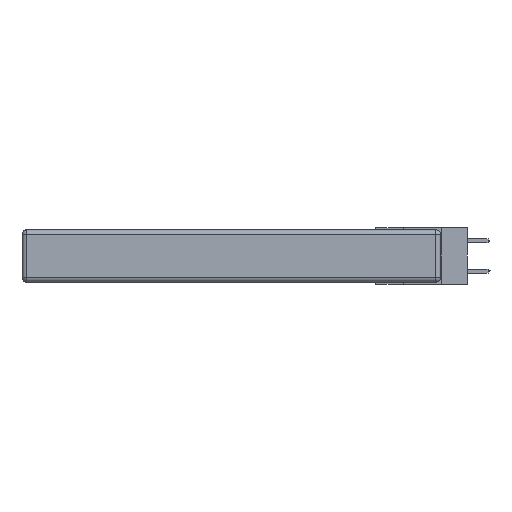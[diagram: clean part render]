
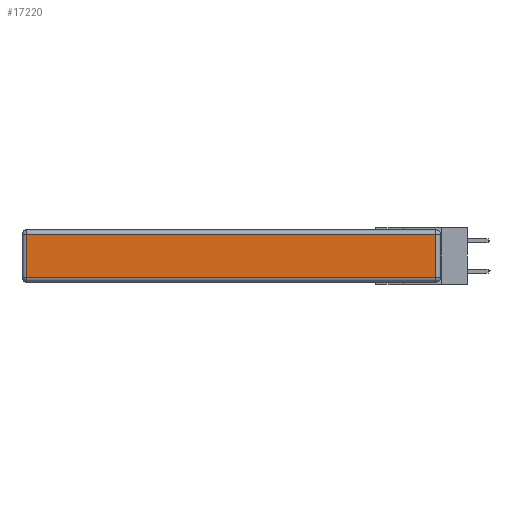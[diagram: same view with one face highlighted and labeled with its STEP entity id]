
A CAD part, left-side view. The second image highlights one B-rep face of the part: STEP entity #17220.
In plain terms, the highlighted planar face has unit normal (-1, 0, 0).
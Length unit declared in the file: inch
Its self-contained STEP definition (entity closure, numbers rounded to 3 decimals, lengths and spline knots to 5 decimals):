
#131 = LINE ( 'NONE', #1619, #1203 ) ;
#206 = CARTESIAN_POINT ( 'NONE',  ( 0., 0., -0.313 ) ) ;
#222 = LINE ( 'NONE', #6790, #11490 ) ;
#1203 = VECTOR ( 'NONE', #11000, 39.37008 ) ;
#1533 = VERTEX_POINT ( 'NONE', #15510 ) ;
#1619 = CARTESIAN_POINT ( 'NONE',  ( 0., 2.75, -0.03 ) ) ;
#1954 = EDGE_CURVE ( 'NONE', #11402, #1533, #14705, .T. ) ;
#1994 = FACE_OUTER_BOUND ( 'NONE', #16047, .T. ) ;
#2025 = LINE ( 'NONE', #206, #3894 ) ;
#3308 = EDGE_CURVE ( 'NONE', #15750, #4034, #222, .T. ) ;
#3894 = VECTOR ( 'NONE', #5530, 39.37008 ) ;
#4034 = VERTEX_POINT ( 'NONE', #7502 ) ;
#4145 = VECTOR ( 'NONE', #9878, 39.37008 ) ;
#5096 = DIRECTION ( 'NONE',  ( 0., 0., 1. ) ) ;
#5530 = DIRECTION ( 'NONE',  ( 0., -1., 0. ) ) ;
#5720 = AXIS2_PLACEMENT_3D ( 'NONE', #16996, #17112, #5096 ) ;
#6790 = CARTESIAN_POINT ( 'NONE',  ( 0., 2.72, -0.343 ) ) ;
#7502 = CARTESIAN_POINT ( 'NONE',  ( 0., 2.72, -0.313 ) ) ;
#7519 = ORIENTED_EDGE ( 'NONE', *, *, #1954, .T. ) ;
#7670 = PLANE ( 'NONE',  #5720 ) ;
#7780 = EDGE_CURVE ( 'NONE', #1533, #15750, #131, .T. ) ;
#8130 = EDGE_CURVE ( 'NONE', #4034, #11402, #2025, .T. ) ;
#9878 = DIRECTION ( 'NONE',  ( 0., 0., 1. ) ) ;
#11000 = DIRECTION ( 'NONE',  ( 0., 1., 0. ) ) ;
#11402 = VERTEX_POINT ( 'NONE', #16280 ) ;
#11416 = CARTESIAN_POINT ( 'NONE',  ( 0., 0.03, -0.343 ) ) ;
#11490 = VECTOR ( 'NONE', #15098, 39.37008 ) ;
#14193 = CARTESIAN_POINT ( 'NONE',  ( 0., 2.72, -0.03 ) ) ;
#14705 = LINE ( 'NONE', #11416, #4145 ) ;
#15098 = DIRECTION ( 'NONE',  ( 0., 0., -1. ) ) ;
#15510 = CARTESIAN_POINT ( 'NONE',  ( 0., 0.03, -0.03 ) ) ;
#15656 = ORIENTED_EDGE ( 'NONE', *, *, #3308, .T. ) ;
#15750 = VERTEX_POINT ( 'NONE', #14193 ) ;
#16047 = EDGE_LOOP ( 'NONE', ( #16347, #7519, #16743, #15656 ) ) ;
#16280 = CARTESIAN_POINT ( 'NONE',  ( 0., 0.03, -0.313 ) ) ;
#16347 = ORIENTED_EDGE ( 'NONE', *, *, #8130, .T. ) ;
#16743 = ORIENTED_EDGE ( 'NONE', *, *, #7780, .T. ) ;
#16996 = CARTESIAN_POINT ( 'NONE',  ( 0., 0., -0.343 ) ) ;
#17112 = DIRECTION ( 'NONE',  ( -1., 0., 0. ) ) ;
#17220 = ADVANCED_FACE ( 'NONE', ( #1994 ), #7670, .T. ) ;
